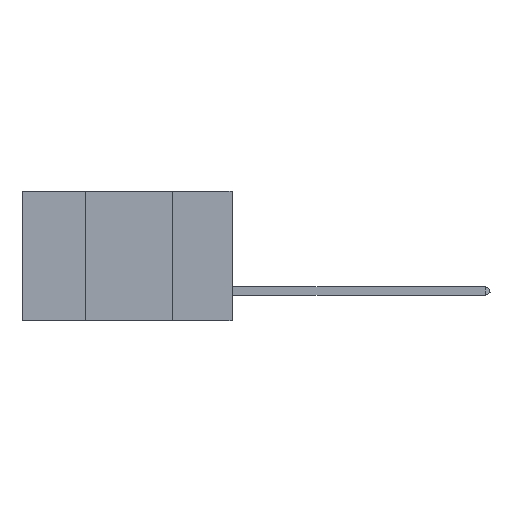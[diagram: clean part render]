
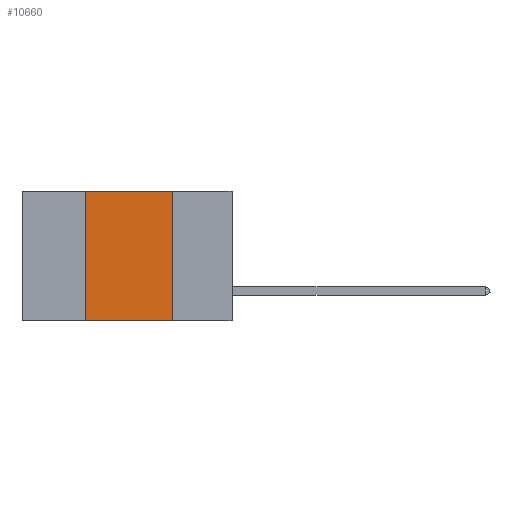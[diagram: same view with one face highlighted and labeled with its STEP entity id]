
A CAD part, left-side view. The second image highlights one B-rep face of the part: STEP entity #10660.
In plain terms, the highlighted planar face has unit normal (-1, 0, 0).
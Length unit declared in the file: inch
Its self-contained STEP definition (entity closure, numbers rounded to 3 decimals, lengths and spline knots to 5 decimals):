
#438 = ORIENTED_EDGE ( 'NONE', *, *, #1396, .F. ) ;
#510 = PLANE ( 'NONE',  #7091 ) ;
#533 = LINE ( 'NONE', #12520, #5441 ) ;
#864 = ORIENTED_EDGE ( 'NONE', *, *, #6569, .F. ) ;
#1184 = CARTESIAN_POINT ( 'NONE',  ( 0., 0.17, 0. ) ) ;
#1396 = EDGE_CURVE ( 'NONE', #3815, #7430, #6518, .T. ) ;
#1489 = DIRECTION ( 'NONE',  ( 0., 0., -1. ) ) ;
#1591 = CARTESIAN_POINT ( 'NONE',  ( 0., 0.6, -0.37 ) ) ;
#2338 = CARTESIAN_POINT ( 'NONE',  ( 0., 0.6, 0. ) ) ;
#2391 = FACE_OUTER_BOUND ( 'NONE', #10496, .T. ) ;
#2438 = ORIENTED_EDGE ( 'NONE', *, *, #9838, .T. ) ;
#2543 = DIRECTION ( 'NONE',  ( 0., -1., 0. ) ) ;
#2958 = ORIENTED_EDGE ( 'NONE', *, *, #5788, .F. ) ;
#3800 = CARTESIAN_POINT ( 'NONE',  ( 0., 0.42, -0.37 ) ) ;
#3815 = VERTEX_POINT ( 'NONE', #9930 ) ;
#4681 = VECTOR ( 'NONE', #8564, 39.37008 ) ;
#5441 = VECTOR ( 'NONE', #11512, 39.37008 ) ;
#5788 = EDGE_CURVE ( 'NONE', #10121, #3815, #10103, .T. ) ;
#6518 = LINE ( 'NONE', #9734, #7256 ) ;
#6569 = EDGE_CURVE ( 'NONE', #7430, #7369, #533, .T. ) ;
#7091 = AXIS2_PLACEMENT_3D ( 'NONE', #2338, #7328, #1489 ) ;
#7256 = VECTOR ( 'NONE', #7693, 39.37008 ) ;
#7328 = DIRECTION ( 'NONE',  ( 1., 0., 0. ) ) ;
#7369 = VERTEX_POINT ( 'NONE', #11384 ) ;
#7430 = VERTEX_POINT ( 'NONE', #1184 ) ;
#7693 = DIRECTION ( 'NONE',  ( 0., -1., 0. ) ) ;
#7750 = LINE ( 'NONE', #1591, #10916 ) ;
#8564 = DIRECTION ( 'NONE',  ( 0., 0., 1. ) ) ;
#9734 = CARTESIAN_POINT ( 'NONE',  ( 0., 0.6, 0. ) ) ;
#9838 = EDGE_CURVE ( 'NONE', #10121, #7369, #7750, .T. ) ;
#9930 = CARTESIAN_POINT ( 'NONE',  ( 0., 0.42, 0. ) ) ;
#10103 = LINE ( 'NONE', #10523, #4681 ) ;
#10121 = VERTEX_POINT ( 'NONE', #3800 ) ;
#10496 = EDGE_LOOP ( 'NONE', ( #864, #438, #2958, #2438 ) ) ;
#10523 = CARTESIAN_POINT ( 'NONE',  ( 0., 0.42, 0. ) ) ;
#10660 = ADVANCED_FACE ( 'NONE', ( #2391 ), #510, .F. ) ;
#10916 = VECTOR ( 'NONE', #2543, 39.37008 ) ;
#11384 = CARTESIAN_POINT ( 'NONE',  ( 0., 0.17, -0.37 ) ) ;
#11512 = DIRECTION ( 'NONE',  ( 0., 0., -1. ) ) ;
#12520 = CARTESIAN_POINT ( 'NONE',  ( 0., 0.17, 0. ) ) ;
